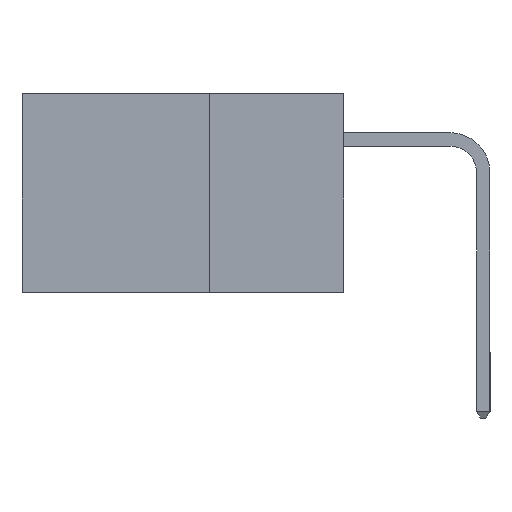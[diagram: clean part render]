
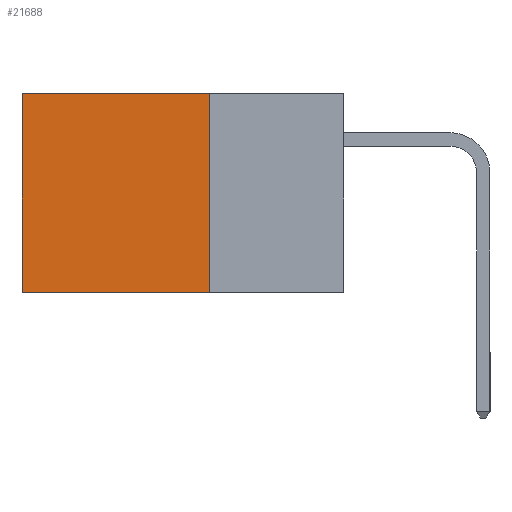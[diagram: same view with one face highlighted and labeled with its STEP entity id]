
A CAD part, left-side view. The second image highlights one B-rep face of the part: STEP entity #21688.
In plain terms, the highlighted planar face has unit normal (-1, 0, 0).
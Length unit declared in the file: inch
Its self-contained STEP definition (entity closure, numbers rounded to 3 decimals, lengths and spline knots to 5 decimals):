
#685 = CARTESIAN_POINT ( 'NONE',  ( 0.298, 0.25, 0. ) ) ;
#723 = VECTOR ( 'NONE', #29130, 39.37008 ) ;
#1671 = EDGE_CURVE ( 'NONE', #19072, #28967, #20576, .T. ) ;
#2638 = ORIENTED_EDGE ( 'NONE', *, *, #1671, .T. ) ;
#3876 = CARTESIAN_POINT ( 'NONE',  ( 0.298, 0.6, 0. ) ) ;
#4416 = CARTESIAN_POINT ( 'NONE',  ( 0.298, 0.6, 0. ) ) ;
#4934 = ORIENTED_EDGE ( 'NONE', *, *, #19335, .F. ) ;
#5249 = VERTEX_POINT ( 'NONE', #12811 ) ;
#5418 = CARTESIAN_POINT ( 'NONE',  ( 0.298, 0.25, 0. ) ) ;
#5690 = LINE ( 'NONE', #18714, #15712 ) ;
#6268 = LINE ( 'NONE', #22135, #23691 ) ;
#6824 = DIRECTION ( 'NONE',  ( 0., 0., -1. ) ) ;
#8487 = EDGE_LOOP ( 'NONE', ( #2638, #13752, #4934, #13978 ) ) ;
#8492 = VERTEX_POINT ( 'NONE', #19790 ) ;
#9642 = LINE ( 'NONE', #5418, #723 ) ;
#10245 = DIRECTION ( 'NONE',  ( 0., 0., -1. ) ) ;
#10829 = FACE_OUTER_BOUND ( 'NONE', #8487, .T. ) ;
#12025 = AXIS2_PLACEMENT_3D ( 'NONE', #685, #26670, #10245 ) ;
#12755 = DIRECTION ( 'NONE',  ( 0., 1., 0. ) ) ;
#12811 = CARTESIAN_POINT ( 'NONE',  ( 0.298, 0.25, -0.37 ) ) ;
#13752 = ORIENTED_EDGE ( 'NONE', *, *, #28339, .F. ) ;
#13978 = ORIENTED_EDGE ( 'NONE', *, *, #28279, .T. ) ;
#15712 = VECTOR ( 'NONE', #25847, 39.37008 ) ;
#17391 = PLANE ( 'NONE',  #12025 ) ;
#18714 = CARTESIAN_POINT ( 'NONE',  ( 0.298, 0.25, 0. ) ) ;
#18727 = VECTOR ( 'NONE', #6824, 39.37008 ) ;
#19072 = VERTEX_POINT ( 'NONE', #3876 ) ;
#19335 = EDGE_CURVE ( 'NONE', #8492, #5249, #5690, .T. ) ;
#19790 = CARTESIAN_POINT ( 'NONE',  ( 0.298, 0.25, 0. ) ) ;
#20576 = LINE ( 'NONE', #4416, #18727 ) ;
#21688 = ADVANCED_FACE ( 'NONE', ( #10829 ), #17391, .F. ) ;
#22135 = CARTESIAN_POINT ( 'NONE',  ( 0.298, 0.25, -0.37 ) ) ;
#23691 = VECTOR ( 'NONE', #12755, 39.37008 ) ;
#25847 = DIRECTION ( 'NONE',  ( 0., 0., -1. ) ) ;
#26670 = DIRECTION ( 'NONE',  ( 1., 0., 0. ) ) ;
#28156 = CARTESIAN_POINT ( 'NONE',  ( 0.298, 0.6, -0.37 ) ) ;
#28279 = EDGE_CURVE ( 'NONE', #8492, #19072, #9642, .T. ) ;
#28339 = EDGE_CURVE ( 'NONE', #5249, #28967, #6268, .T. ) ;
#28967 = VERTEX_POINT ( 'NONE', #28156 ) ;
#29130 = DIRECTION ( 'NONE',  ( 0., 1., 0. ) ) ;
